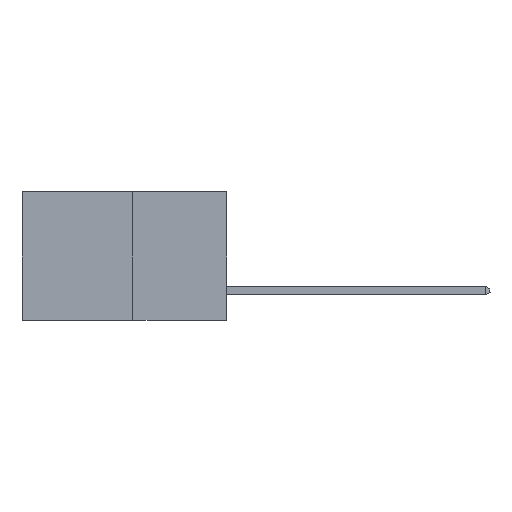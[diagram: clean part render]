
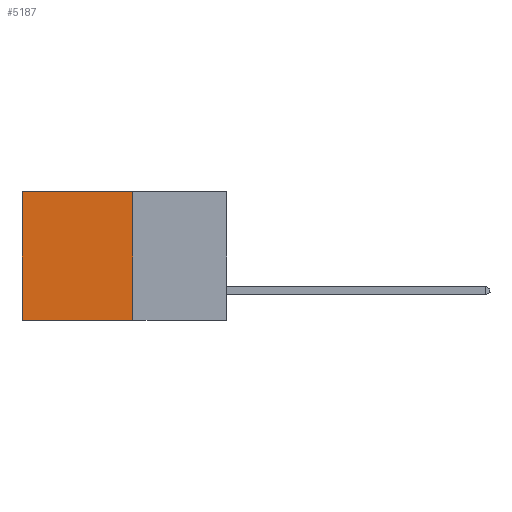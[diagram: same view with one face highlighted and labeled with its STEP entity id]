
A CAD part, left-side view. The second image highlights one B-rep face of the part: STEP entity #5187.
In plain terms, the highlighted planar face has unit normal (-1, 0, 0).
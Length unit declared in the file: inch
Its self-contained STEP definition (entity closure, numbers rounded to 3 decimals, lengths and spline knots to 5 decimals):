
#505 = EDGE_CURVE ( 'NONE', #16573, #4828, #8115, .T. ) ;
#1611 = VECTOR ( 'NONE', #10321, 39.37008 ) ;
#1622 = FACE_OUTER_BOUND ( 'NONE', #15152, .T. ) ;
#3841 = LINE ( 'NONE', #25416, #9593 ) ;
#3932 = CARTESIAN_POINT ( 'NONE',  ( 0.277, 0.59, -0.37 ) ) ;
#4828 = VERTEX_POINT ( 'NONE', #22933 ) ;
#5187 = ADVANCED_FACE ( 'NONE', ( #1622 ), #18652, .F. ) ;
#5201 = VECTOR ( 'NONE', #23770, 39.37008 ) ;
#5681 = AXIS2_PLACEMENT_3D ( 'NONE', #18511, #18483, #18474 ) ;
#5688 = ORIENTED_EDGE ( 'NONE', *, *, #16364, .F. ) ;
#6194 = DIRECTION ( 'NONE',  ( 0., 1., 0. ) ) ;
#8115 = LINE ( 'NONE', #22657, #18100 ) ;
#9593 = VECTOR ( 'NONE', #21274, 39.37008 ) ;
#9759 = CARTESIAN_POINT ( 'NONE',  ( 0.277, 0.27, -0.37 ) ) ;
#10321 = DIRECTION ( 'NONE',  ( 0., 0., -1. ) ) ;
#11517 = LINE ( 'NONE', #25842, #5201 ) ;
#11907 = VERTEX_POINT ( 'NONE', #14531 ) ;
#13744 = LINE ( 'NONE', #3932, #1611 ) ;
#14199 = ORIENTED_EDGE ( 'NONE', *, *, #22447, .T. ) ;
#14531 = CARTESIAN_POINT ( 'NONE',  ( 0.277, 0.27, 0. ) ) ;
#15152 = EDGE_LOOP ( 'NONE', ( #14199, #22085, #5688, #24533 ) ) ;
#15557 = EDGE_CURVE ( 'NONE', #11907, #17180, #3841, .T. ) ;
#16364 = EDGE_CURVE ( 'NONE', #11907, #16573, #11517, .T. ) ;
#16573 = VERTEX_POINT ( 'NONE', #9759 ) ;
#17180 = VERTEX_POINT ( 'NONE', #20470 ) ;
#18100 = VECTOR ( 'NONE', #6194, 39.37008 ) ;
#18474 = DIRECTION ( 'NONE',  ( 0., 0., -1. ) ) ;
#18483 = DIRECTION ( 'NONE',  ( 1., 0., 0. ) ) ;
#18511 = CARTESIAN_POINT ( 'NONE',  ( 0.277, 0.27, -0.37 ) ) ;
#18652 = PLANE ( 'NONE',  #5681 ) ;
#20470 = CARTESIAN_POINT ( 'NONE',  ( 0.277, 0.59, 0. ) ) ;
#21274 = DIRECTION ( 'NONE',  ( 0., 1., 0. ) ) ;
#22085 = ORIENTED_EDGE ( 'NONE', *, *, #505, .F. ) ;
#22447 = EDGE_CURVE ( 'NONE', #17180, #4828, #13744, .T. ) ;
#22657 = CARTESIAN_POINT ( 'NONE',  ( 0.277, 0.27, -0.37 ) ) ;
#22933 = CARTESIAN_POINT ( 'NONE',  ( 0.277, 0.59, -0.37 ) ) ;
#23770 = DIRECTION ( 'NONE',  ( 0., 0., -1. ) ) ;
#24533 = ORIENTED_EDGE ( 'NONE', *, *, #15557, .T. ) ;
#25416 = CARTESIAN_POINT ( 'NONE',  ( 0.277, 0.27, 0. ) ) ;
#25842 = CARTESIAN_POINT ( 'NONE',  ( 0.277, 0.27, -0.37 ) ) ;
